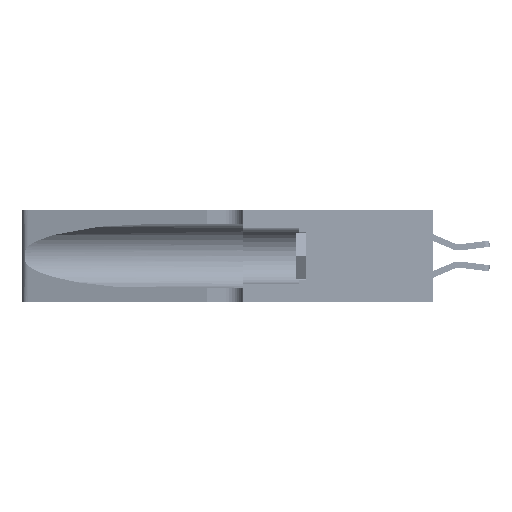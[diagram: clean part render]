
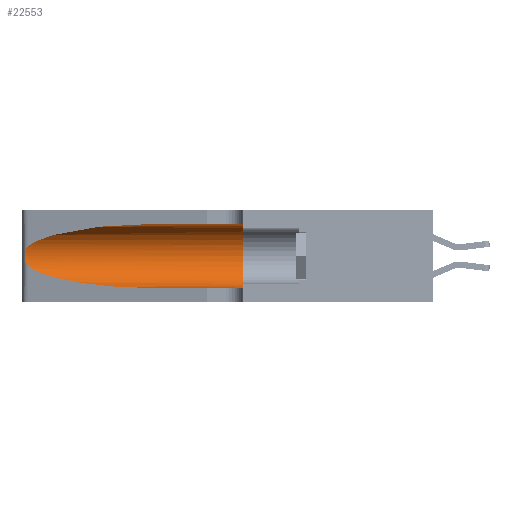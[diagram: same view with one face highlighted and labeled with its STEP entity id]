
A CAD part, left-side view. The second image highlights one B-rep face of the part: STEP entity #22553.
In plain terms, the highlighted cylindrical face has radius 3.308 mm (diameter 6.617 mm), a partial arc.
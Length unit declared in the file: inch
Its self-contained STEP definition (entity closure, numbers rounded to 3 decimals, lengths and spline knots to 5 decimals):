
#6545 = VERTEX_POINT ( 'NONE', #37624 ) ;
#6860 = ORIENTED_EDGE ( 'NONE', *, *, #19224, .F. ) ;
#7877 = CARTESIAN_POINT ( 'NONE',  ( 0.1305, 0.35, 0.05475 ) ) ;
#8030 = ORIENTED_EDGE ( 'NONE', *, *, #17348, .T. ) ;
#8611 = CARTESIAN_POINT ( 'NONE',  ( 0.1305, 0.72297, 0.05475 ) ) ;
#9379 = CARTESIAN_POINT ( 'NONE',  ( 0.25555, 1.22994, 0.2215 ) ) ;
#9701 = CARTESIAN_POINT ( 'NONE',  ( 0.25487, 1.22718, 0.22369 ) ) ;
#10208 = CARTESIAN_POINT ( 'NONE',  ( 0.25487, 1.22718, 0.14631 ) ) ;
#10719 = CARTESIAN_POINT ( 'NONE',  ( 0.25856, 1.23593, 0.16098 ) ) ;
#11168 = CARTESIAN_POINT ( 'NONE',  ( 0.25487, 1.22718, 0.14631 ) ) ;
#11277 = B_SPLINE_CURVE_WITH_KNOTS ( 'NONE', 3,
 ( #9701, #9379, #13870, #48729, #37300, #25082, #32994, #21594, #49246, #10719, #41779, #37654, #37808, #10208 ),
 .UNSPECIFIED., .F., .F.,
 ( 4, 2, 2, 2, 2, 2, 4 ),
 ( 0., 0.00027, 0.00053, 0.00107, 0.0016, 0.00187, 0.00214 ),
 .UNSPECIFIED. ) ;
#11288 = EDGE_LOOP ( 'NONE', ( #45239, #50002, #49719, #8030, #6860, #28311 ) ) ;
#11744 = CARTESIAN_POINT ( 'NONE',  ( 0.1305, 1.61858, 0.05475 ) ) ;
#13641 = AXIS2_PLACEMENT_3D ( 'NONE', #30205, #22094, #18303 ) ;
#13870 = CARTESIAN_POINT ( 'NONE',  ( 0.25639, 1.23184, 0.21858 ) ) ;
#13877 = AXIS2_PLACEMENT_3D ( 'NONE', #35216, #15563, #43335 ) ;
#14345 = CIRCLE ( 'NONE', #13877, 0.13025 ) ;
#15563 = DIRECTION ( 'NONE',  ( 0., 1., 0. ) ) ;
#15626 = EDGE_CURVE ( 'NONE', #21319, #25342, #47335, .T. ) ;
#16072 = DIRECTION ( 'NONE',  ( 0., -1., 0. ) ) ;
#17036 = EDGE_CURVE ( 'NONE', #46244, #21319, #11277, .T. ) ;
#17348 = EDGE_CURVE ( 'NONE', #25342, #43074, #32491, .T. ) ;
#17667 = CARTESIAN_POINT ( 'NONE',  ( 0.18966, 0.96281, 0.31525 ) ) ;
#17846 = CARTESIAN_POINT ( 'NONE',  ( 0.25487, 1.22718, 0.22369 ) ) ;
#18303 = DIRECTION ( 'NONE',  ( 0., 0., -1. ) ) ;
#19224 = EDGE_CURVE ( 'NONE', #51006, #43074, #14345, .T. ) ;
#20675 = DIRECTION ( 'NONE',  ( 0., -1., 0. ) ) ;
#21319 = VERTEX_POINT ( 'NONE', #11168 ) ;
#21594 = CARTESIAN_POINT ( 'NONE',  ( 0.26075, 1.23896, 0.178 ) ) ;
#21983 = VECTOR ( 'NONE', #16072, 39.37008 ) ;
#22094 = DIRECTION ( 'NONE',  ( 0., -1., 0. ) ) ;
#22553 = ADVANCED_FACE ( 'NONE', ( #44754 ), #23754, .F. ) ;
#23510 = VECTOR ( 'NONE', #20675, 39.37008 ) ;
#23754 = CYLINDRICAL_SURFACE ( 'NONE', #13641, 0.13025 ) ;
#24321 = CARTESIAN_POINT ( 'NONE',  ( 0.2373, 1.15595, 0.08982 ) ) ;
#24848 = CARTESIAN_POINT ( 'NONE',  ( 0.25487, 1.22718, 0.22369 ) ) ;
#25082 = CARTESIAN_POINT ( 'NONE',  ( 0.26018, 1.23835, 0.19895 ) ) ;
#25342 = VERTEX_POINT ( 'NONE', #45707 ) ;
#28108 = CARTESIAN_POINT ( 'NONE',  ( 0.25487, 1.22718, 0.14631 ) ) ;
#28265 = CARTESIAN_POINT ( 'NONE',  ( 0.18966, 0.96281, 0.05475 ) ) ;
#28311 = ORIENTED_EDGE ( 'NONE', *, *, #42333, .F. ) ;
#29061 = CARTESIAN_POINT ( 'NONE',  ( 0.2373, 1.15595, 0.28018 ) ) ;
#30205 = CARTESIAN_POINT ( 'NONE',  ( 0.1305, 1.61858, 0.185 ) ) ;
#32491 = LINE ( 'NONE', #11744, #21983 ) ;
#32602 = CARTESIAN_POINT ( 'NONE',  ( 0.1305, 1.61858, 0.31525 ) ) ;
#32994 = CARTESIAN_POINT ( 'NONE',  ( 0.26075, 1.23896, 0.19203 ) ) ;
#35216 = CARTESIAN_POINT ( 'NONE',  ( 0.1305, 0.35, 0.185 ) ) ;
#35236 = LINE ( 'NONE', #32602, #23510 ) ;
#35534 = EDGE_CURVE ( 'NONE', #6545, #46244, #38156, .T. ) ;
#37300 = CARTESIAN_POINT ( 'NONE',  ( 0.25854, 1.2359, 0.20912 ) ) ;
#37624 = CARTESIAN_POINT ( 'NONE',  ( 0.1305, 0.72297, 0.31525 ) ) ;
#37654 = CARTESIAN_POINT ( 'NONE',  ( 0.25639, 1.23186, 0.15144 ) ) ;
#37808 = CARTESIAN_POINT ( 'NONE',  ( 0.25555, 1.22993, 0.14849 ) ) ;
#38156 =( BOUNDED_CURVE ( )  B_SPLINE_CURVE ( 3, ( #40791, #17667, #29061, #17846 ),
 .UNSPECIFIED., .F., .F. ) 
 B_SPLINE_CURVE_WITH_KNOTS ( ( 4, 4 ),
 ( 1.5708, 2.84003 ),
 .UNSPECIFIED. ) 
 CURVE ( )  GEOMETRIC_REPRESENTATION_ITEM ( )  RATIONAL_B_SPLINE_CURVE ( ( 1., 0.87, 0.87, 1. ) ) 
 REPRESENTATION_ITEM ( '' )  );
#40791 = CARTESIAN_POINT ( 'NONE',  ( 0.1305, 0.72297, 0.31525 ) ) ;
#41779 = CARTESIAN_POINT ( 'NONE',  ( 0.25789, 1.23486, 0.15765 ) ) ;
#42333 = EDGE_CURVE ( 'NONE', #6545, #51006, #35236, .T. ) ;
#43074 = VERTEX_POINT ( 'NONE', #7877 ) ;
#43335 = DIRECTION ( 'NONE',  ( 0., 0., 1. ) ) ;
#44754 = FACE_OUTER_BOUND ( 'NONE', #11288, .T. ) ;
#45239 = ORIENTED_EDGE ( 'NONE', *, *, #35534, .T. ) ;
#45707 = CARTESIAN_POINT ( 'NONE',  ( 0.1305, 0.72297, 0.05475 ) ) ;
#46244 = VERTEX_POINT ( 'NONE', #24848 ) ;
#47335 =( BOUNDED_CURVE ( )  B_SPLINE_CURVE ( 3, ( #28108, #24321, #28265, #8611 ),
 .UNSPECIFIED., .F., .T. ) 
 B_SPLINE_CURVE_WITH_KNOTS ( ( 4, 4 ),
 ( 3.44316, 4.71239 ),
 .UNSPECIFIED. ) 
 CURVE ( )  GEOMETRIC_REPRESENTATION_ITEM ( )  RATIONAL_B_SPLINE_CURVE ( ( 1., 0.87, 0.87, 1. ) ) 
 REPRESENTATION_ITEM ( '' )  );
#47893 = CARTESIAN_POINT ( 'NONE',  ( 0.1305, 0.35, 0.31525 ) ) ;
#48729 = CARTESIAN_POINT ( 'NONE',  ( 0.25787, 1.23484, 0.2124 ) ) ;
#49246 = CARTESIAN_POINT ( 'NONE',  ( 0.26017, 1.23833, 0.17102 ) ) ;
#49719 = ORIENTED_EDGE ( 'NONE', *, *, #15626, .T. ) ;
#50002 = ORIENTED_EDGE ( 'NONE', *, *, #17036, .T. ) ;
#51006 = VERTEX_POINT ( 'NONE', #47893 ) ;
